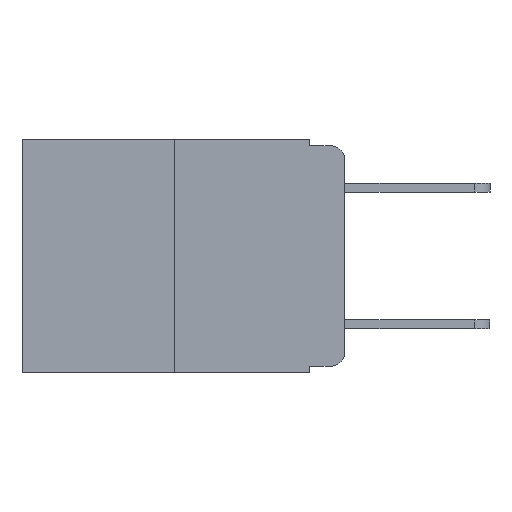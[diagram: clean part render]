
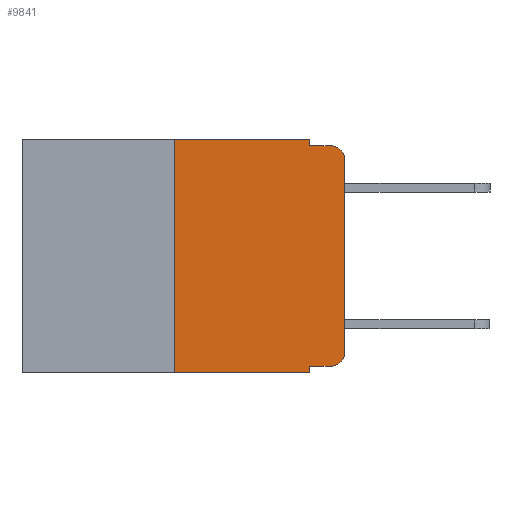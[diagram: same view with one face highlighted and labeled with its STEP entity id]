
A CAD part, left-side view. The second image highlights one B-rep face of the part: STEP entity #9841.
In plain terms, the highlighted planar face has unit normal (-1, 0, 0).
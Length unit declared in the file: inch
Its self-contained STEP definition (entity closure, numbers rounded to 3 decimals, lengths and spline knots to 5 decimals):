
#201 = CARTESIAN_POINT ( 'NONE',  ( 0., 0.051, -0.343 ) ) ;
#444 = CARTESIAN_POINT ( 'NONE',  ( 0., 0.051, 0. ) ) ;
#564 = DIRECTION ( 'NONE',  ( 0., -1., 0. ) ) ;
#612 = ORIENTED_EDGE ( 'NONE', *, *, #1578, .F. ) ;
#722 = CARTESIAN_POINT ( 'NONE',  ( 0., 0.473, 0. ) ) ;
#764 = EDGE_CURVE ( 'NONE', #10366, #1834, #6539, .T. ) ;
#784 = DIRECTION ( 'NONE',  ( -1., 0., 0. ) ) ;
#903 = VECTOR ( 'NONE', #3889, 39.37008 ) ;
#1133 = CARTESIAN_POINT ( 'NONE',  ( 0., 0., -0.313 ) ) ;
#1561 = EDGE_LOOP ( 'NONE', ( #2121, #3418, #612, #1710, #2107, #2463, #2555, #3616, #3905, #3951 ) ) ;
#1578 = EDGE_CURVE ( 'NONE', #11750, #1834, #6805, .T. ) ;
#1710 = ORIENTED_EDGE ( 'NONE', *, *, #3847, .F. ) ;
#1744 = VECTOR ( 'NONE', #8773, 39.37008 ) ;
#1834 = VERTEX_POINT ( 'NONE', #7652 ) ;
#2083 = VERTEX_POINT ( 'NONE', #8981 ) ;
#2107 = ORIENTED_EDGE ( 'NONE', *, *, #10776, .F. ) ;
#2121 = ORIENTED_EDGE ( 'NONE', *, *, #12231, .T. ) ;
#2463 = ORIENTED_EDGE ( 'NONE', *, *, #7761, .F. ) ;
#2555 = ORIENTED_EDGE ( 'NONE', *, *, #9669, .T. ) ;
#3218 = CARTESIAN_POINT ( 'NONE',  ( 0., 0., -0.03 ) ) ;
#3418 = ORIENTED_EDGE ( 'NONE', *, *, #764, .T. ) ;
#3616 = ORIENTED_EDGE ( 'NONE', *, *, #8371, .F. ) ;
#3825 = VECTOR ( 'NONE', #12525, 39.37008 ) ;
#3847 = EDGE_CURVE ( 'NONE', #8262, #11750, #4301, .T. ) ;
#3885 = VERTEX_POINT ( 'NONE', #10599 ) ;
#3889 = DIRECTION ( 'NONE',  ( 0., 0., -1. ) ) ;
#3905 = ORIENTED_EDGE ( 'NONE', *, *, #9670, .T. ) ;
#3931 = DIRECTION ( 'NONE',  ( 0., 0., 1. ) ) ;
#3951 = ORIENTED_EDGE ( 'NONE', *, *, #12026, .T. ) ;
#4251 = VERTEX_POINT ( 'NONE', #1133 ) ;
#4301 = LINE ( 'NONE', #11402, #903 ) ;
#4321 = DIRECTION ( 'NONE',  ( -1., 0., 0. ) ) ;
#4585 = VERTEX_POINT ( 'NONE', #5024 ) ;
#4703 = AXIS2_PLACEMENT_3D ( 'NONE', #10030, #4321, #10908 ) ;
#5024 = CARTESIAN_POINT ( 'NONE',  ( 0., 0.25, 0. ) ) ;
#5093 = VECTOR ( 'NONE', #10584, 39.37008 ) ;
#5196 = PLANE ( 'NONE',  #8290 ) ;
#5770 = CARTESIAN_POINT ( 'NONE',  ( 0., 0.051, -0.01 ) ) ;
#6138 = CARTESIAN_POINT ( 'NONE',  ( 0., 0.02, -0.333 ) ) ;
#6452 = LINE ( 'NONE', #722, #3825 ) ;
#6511 = VECTOR ( 'NONE', #10134, 39.37008 ) ;
#6539 = CIRCLE ( 'NONE', #10999, 0.02 ) ;
#6805 = LINE ( 'NONE', #12715, #6511 ) ;
#7112 = DIRECTION ( 'NONE',  ( 0., 0., -1. ) ) ;
#7499 = VECTOR ( 'NONE', #3931, 39.37008 ) ;
#7591 = VERTEX_POINT ( 'NONE', #201 ) ;
#7652 = CARTESIAN_POINT ( 'NONE',  ( 0., 0.02, -0.01 ) ) ;
#7761 = EDGE_CURVE ( 'NONE', #3885, #4585, #12327, .T. ) ;
#8262 = VERTEX_POINT ( 'NONE', #10391 ) ;
#8290 = AXIS2_PLACEMENT_3D ( 'NONE', #11685, #12561, #7112 ) ;
#8371 = EDGE_CURVE ( 'NONE', #2083, #7591, #10413, .T. ) ;
#8773 = DIRECTION ( 'NONE',  ( 0., -1., 0. ) ) ;
#8981 = CARTESIAN_POINT ( 'NONE',  ( 0., 0.051, -0.333 ) ) ;
#9451 = VECTOR ( 'NONE', #564, 39.37008 ) ;
#9669 = EDGE_CURVE ( 'NONE', #3885, #7591, #9738, .T. ) ;
#9670 = EDGE_CURVE ( 'NONE', #2083, #10801, #12076, .T. ) ;
#9696 = CARTESIAN_POINT ( 'NONE',  ( 0., 0.25, 0. ) ) ;
#9738 = LINE ( 'NONE', #10634, #1744 ) ;
#9841 = ADVANCED_FACE ( 'NONE', ( #10437 ), #5196, .F. ) ;
#10030 = CARTESIAN_POINT ( 'NONE',  ( 0., 0.02, -0.313 ) ) ;
#10098 = VECTOR ( 'NONE', #11170, 39.37008 ) ;
#10134 = DIRECTION ( 'NONE',  ( 0., -1., 0. ) ) ;
#10239 = CIRCLE ( 'NONE', #4703, 0.02 ) ;
#10298 = CARTESIAN_POINT ( 'NONE',  ( 0., 0., 0. ) ) ;
#10366 = VERTEX_POINT ( 'NONE', #3218 ) ;
#10376 = LINE ( 'NONE', #10298, #10098 ) ;
#10391 = CARTESIAN_POINT ( 'NONE',  ( 0., 0.051, 0. ) ) ;
#10413 = LINE ( 'NONE', #444, #5093 ) ;
#10437 = FACE_OUTER_BOUND ( 'NONE', #1561, .T. ) ;
#10584 = DIRECTION ( 'NONE',  ( 0., 0., -1. ) ) ;
#10599 = CARTESIAN_POINT ( 'NONE',  ( 0., 0.25, -0.343 ) ) ;
#10634 = CARTESIAN_POINT ( 'NONE',  ( 0., 0.473, -0.343 ) ) ;
#10776 = EDGE_CURVE ( 'NONE', #4585, #8262, #6452, .T. ) ;
#10801 = VERTEX_POINT ( 'NONE', #6138 ) ;
#10908 = DIRECTION ( 'NONE',  ( 0., 0., -1. ) ) ;
#10999 = AXIS2_PLACEMENT_3D ( 'NONE', #12471, #784, #11752 ) ;
#11170 = DIRECTION ( 'NONE',  ( 0., 0., 1. ) ) ;
#11402 = CARTESIAN_POINT ( 'NONE',  ( 0., 0.051, 0. ) ) ;
#11685 = CARTESIAN_POINT ( 'NONE',  ( 0., 0.473, 0. ) ) ;
#11750 = VERTEX_POINT ( 'NONE', #5770 ) ;
#11752 = DIRECTION ( 'NONE',  ( 0., 0., -1. ) ) ;
#12026 = EDGE_CURVE ( 'NONE', #10801, #4251, #10239, .T. ) ;
#12076 = LINE ( 'NONE', #12371, #9451 ) ;
#12231 = EDGE_CURVE ( 'NONE', #4251, #10366, #10376, .T. ) ;
#12327 = LINE ( 'NONE', #9696, #7499 ) ;
#12371 = CARTESIAN_POINT ( 'NONE',  ( 0., 0.051, -0.333 ) ) ;
#12471 = CARTESIAN_POINT ( 'NONE',  ( 0., 0.02, -0.03 ) ) ;
#12525 = DIRECTION ( 'NONE',  ( 0., -1., 0. ) ) ;
#12561 = DIRECTION ( 'NONE',  ( 1., 0., 0. ) ) ;
#12715 = CARTESIAN_POINT ( 'NONE',  ( 0., 0.051, -0.01 ) ) ;
